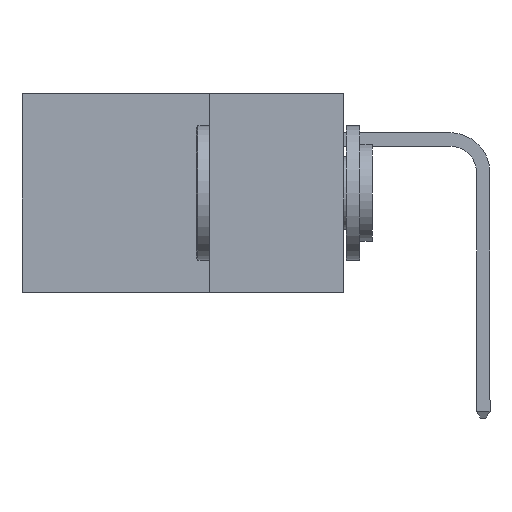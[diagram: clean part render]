
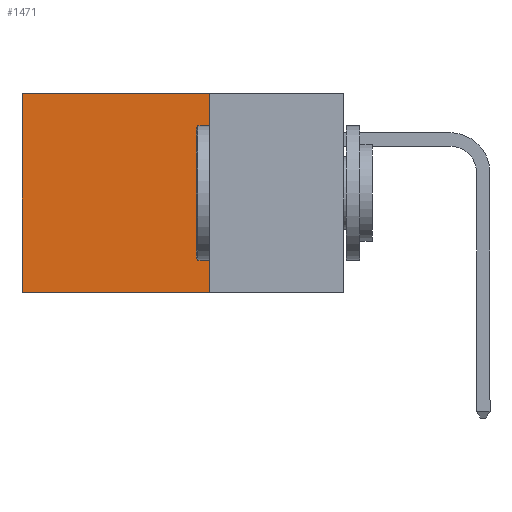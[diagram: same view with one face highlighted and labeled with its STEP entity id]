
A CAD part, left-side view. The second image highlights one B-rep face of the part: STEP entity #1471.
In plain terms, the highlighted planar face has unit normal (-1, 0, 0).
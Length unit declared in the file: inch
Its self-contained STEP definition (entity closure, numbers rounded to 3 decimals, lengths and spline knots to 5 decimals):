
#4 = ORIENTED_EDGE ( 'NONE', *, *, #7251, .F. ) ;
#88 = CARTESIAN_POINT ( 'NONE',  ( 0.2615, 0.25, -0.37 ) ) ;
#1247 = FACE_OUTER_BOUND ( 'NONE', #8080, .T. ) ;
#1283 = CARTESIAN_POINT ( 'NONE',  ( 0.2615, 0.6, 0. ) ) ;
#1471 = ADVANCED_FACE ( 'NONE', ( #1247 ), #8341, .F. ) ;
#1585 = VERTEX_POINT ( 'NONE', #1283 ) ;
#1890 = CARTESIAN_POINT ( 'NONE',  ( 0.2615, 0.25, -0.37 ) ) ;
#2039 = CARTESIAN_POINT ( 'NONE',  ( 0.2615, 0.25, -0.37 ) ) ;
#2374 = VERTEX_POINT ( 'NONE', #88 ) ;
#2607 = DIRECTION ( 'NONE',  ( 0., 0., -1. ) ) ;
#2712 = VECTOR ( 'NONE', #6677, 39.37008 ) ;
#2952 = LINE ( 'NONE', #1890, #2712 ) ;
#3026 = DIRECTION ( 'NONE',  ( 0., 1., 0. ) ) ;
#4039 = EDGE_CURVE ( 'NONE', #2374, #4277, #2952, .T. ) ;
#4277 = VERTEX_POINT ( 'NONE', #4460 ) ;
#4458 = VERTEX_POINT ( 'NONE', #7832 ) ;
#4460 = CARTESIAN_POINT ( 'NONE',  ( 0.2615, 0.6, -0.37 ) ) ;
#4467 = VECTOR ( 'NONE', #6997, 39.37008 ) ;
#5427 = LINE ( 'NONE', #8110, #6961 ) ;
#5843 = CARTESIAN_POINT ( 'NONE',  ( 0.2615, 0.25, 0. ) ) ;
#6018 = AXIS2_PLACEMENT_3D ( 'NONE', #8995, #6960, #7411 ) ;
#6090 = LINE ( 'NONE', #2039, #4467 ) ;
#6215 = LINE ( 'NONE', #5843, #7732 ) ;
#6223 = EDGE_CURVE ( 'NONE', #4458, #1585, #6215, .T. ) ;
#6677 = DIRECTION ( 'NONE',  ( 0., 1., 0. ) ) ;
#6857 = ORIENTED_EDGE ( 'NONE', *, *, #4039, .F. ) ;
#6960 = DIRECTION ( 'NONE',  ( 1., 0., 0. ) ) ;
#6961 = VECTOR ( 'NONE', #2607, 39.37008 ) ;
#6997 = DIRECTION ( 'NONE',  ( 0., 0., -1. ) ) ;
#7251 = EDGE_CURVE ( 'NONE', #4458, #2374, #6090, .T. ) ;
#7411 = DIRECTION ( 'NONE',  ( 0., 0., -1. ) ) ;
#7427 = ORIENTED_EDGE ( 'NONE', *, *, #9005, .T. ) ;
#7732 = VECTOR ( 'NONE', #3026, 39.37008 ) ;
#7740 = ORIENTED_EDGE ( 'NONE', *, *, #6223, .T. ) ;
#7832 = CARTESIAN_POINT ( 'NONE',  ( 0.2615, 0.25, 0. ) ) ;
#8080 = EDGE_LOOP ( 'NONE', ( #7427, #6857, #4, #7740 ) ) ;
#8110 = CARTESIAN_POINT ( 'NONE',  ( 0.2615, 0.6, -0.37 ) ) ;
#8341 = PLANE ( 'NONE',  #6018 ) ;
#8995 = CARTESIAN_POINT ( 'NONE',  ( 0.2615, 0.25, -0.37 ) ) ;
#9005 = EDGE_CURVE ( 'NONE', #1585, #4277, #5427, .T. ) ;
